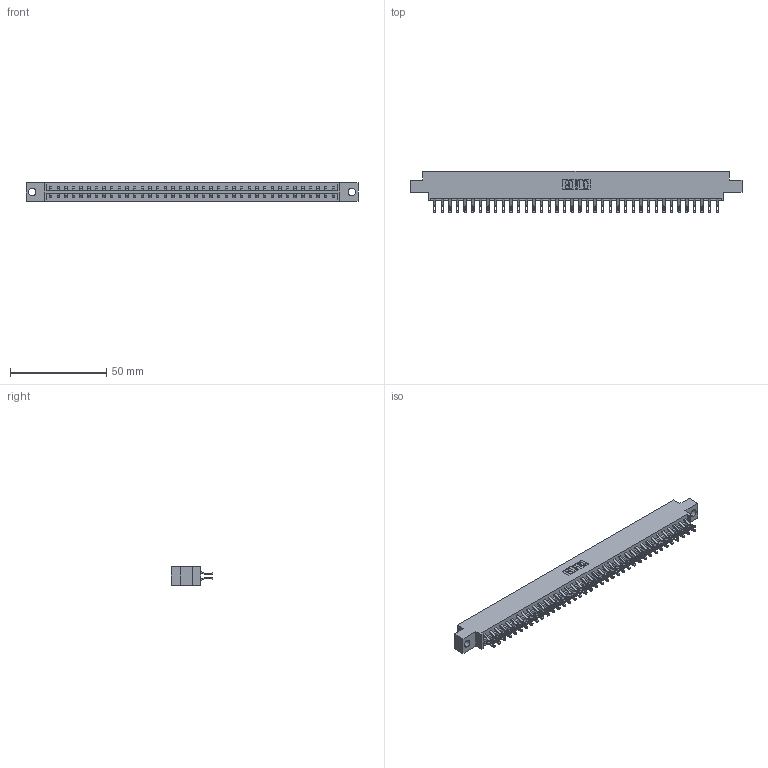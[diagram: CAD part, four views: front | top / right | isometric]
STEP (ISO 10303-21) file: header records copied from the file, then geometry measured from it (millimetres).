
FILE_DESCRIPTION (( 'STEP AP203' ), '1' );
FILE_NAME ('833-076-555-804.STEP', '2020-06-05T18:49:56', ( '' ), ( '' ), 'SwSTEP 2.0', 'SolidWorks 2020', '' );
FILE_SCHEMA (( 'CONFIG_CONTROL_DESIGN' ));
Length unit declared in the file: inch
Products named in the file (3): 345-292-001_555 Tail; 833-076-555-804; 833 Part_Offset - .156 Dia - TH
Assembly tree (77 placements, depth 2):
  833-076-555-804
    833 Part_Offset - .156 Dia - TH
    345-292-001_555 Tail  x76
Bounding box: 172.11 x 21.47 x 9.4 mm (x, y, z)
Volume: 17438.9 mm3; surface area: 21418.8 mm2
Topology: 77 solids, 77 shells, 4526 faces, 14231 edges, 9486 vertices
Faces by surface type: plane 2658, cylinder 1868
Entity records: 25425 total; most frequent: CARTESIAN_POINT 4256, ORIENTED_EDGE 4162, DIRECTION 3613, EDGE_CURVE 2081, LINE 1933, VECTOR 1933, VERTEX_POINT 1386, AXIS2_PLACEMENT_3D 840
